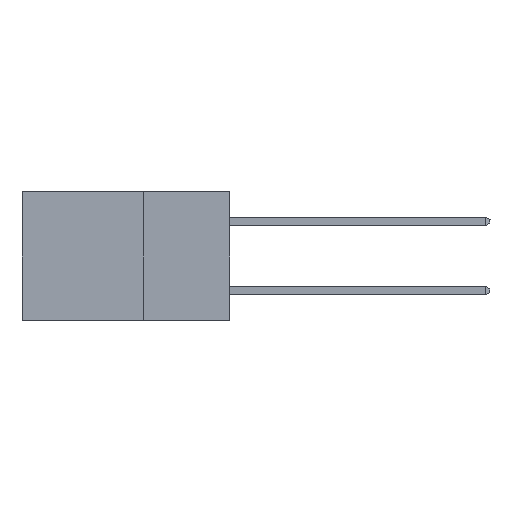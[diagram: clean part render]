
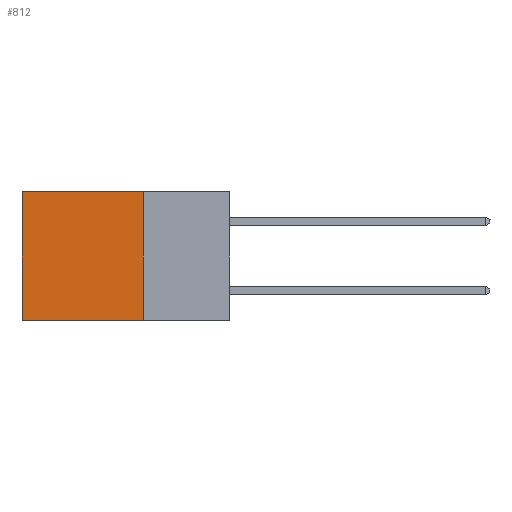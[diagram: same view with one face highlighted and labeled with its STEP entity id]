
A CAD part, left-side view. The second image highlights one B-rep face of the part: STEP entity #812.
In plain terms, the highlighted planar face has unit normal (-1, 0, 0).
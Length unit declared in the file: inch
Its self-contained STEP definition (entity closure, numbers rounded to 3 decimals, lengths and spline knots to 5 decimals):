
#155 = AXIS2_PLACEMENT_3D ( 'NONE', #5176, #6276, #11299 ) ;
#812 = ADVANCED_FACE ( 'NONE', ( #1641 ), #8886, .F. ) ;
#845 = ORIENTED_EDGE ( 'NONE', *, *, #6398, .T. ) ;
#1244 = CARTESIAN_POINT ( 'NONE',  ( 0.2615, 0.25, -0.37 ) ) ;
#1265 = VECTOR ( 'NONE', #4782, 39.37008 ) ;
#1641 = FACE_OUTER_BOUND ( 'NONE', #13665, .T. ) ;
#1705 = CARTESIAN_POINT ( 'NONE',  ( 0.2615, 0.6, -0.37 ) ) ;
#1787 = VERTEX_POINT ( 'NONE', #9597 ) ;
#1824 = LINE ( 'NONE', #1244, #1265 ) ;
#2248 = ORIENTED_EDGE ( 'NONE', *, *, #15168, .T. ) ;
#2853 = VERTEX_POINT ( 'NONE', #4912 ) ;
#3086 = DIRECTION ( 'NONE',  ( 0., 1., 0. ) ) ;
#3244 = CARTESIAN_POINT ( 'NONE',  ( 0.2615, 0.25, -0.37 ) ) ;
#3305 = VECTOR ( 'NONE', #6495, 39.37008 ) ;
#3324 = LINE ( 'NONE', #15288, #11066 ) ;
#3363 = CARTESIAN_POINT ( 'NONE',  ( 0.2615, 0.25, 0. ) ) ;
#4782 = DIRECTION ( 'NONE',  ( 0., 0., -1. ) ) ;
#4912 = CARTESIAN_POINT ( 'NONE',  ( 0.2615, 0.6, -0.37 ) ) ;
#5126 = EDGE_CURVE ( 'NONE', #6088, #2853, #5587, .T. ) ;
#5176 = CARTESIAN_POINT ( 'NONE',  ( 0.2615, 0.25, -0.37 ) ) ;
#5587 = LINE ( 'NONE', #3244, #8245 ) ;
#6088 = VERTEX_POINT ( 'NONE', #9247 ) ;
#6276 = DIRECTION ( 'NONE',  ( 1., 0., 0. ) ) ;
#6398 = EDGE_CURVE ( 'NONE', #13326, #1787, #3324, .T. ) ;
#6495 = DIRECTION ( 'NONE',  ( 0., 0., -1. ) ) ;
#8245 = VECTOR ( 'NONE', #3086, 39.37008 ) ;
#8886 = PLANE ( 'NONE',  #155 ) ;
#9247 = CARTESIAN_POINT ( 'NONE',  ( 0.2615, 0.25, -0.37 ) ) ;
#9597 = CARTESIAN_POINT ( 'NONE',  ( 0.2615, 0.6, 0. ) ) ;
#9731 = LINE ( 'NONE', #1705, #3305 ) ;
#11066 = VECTOR ( 'NONE', #12883, 39.37008 ) ;
#11299 = DIRECTION ( 'NONE',  ( 0., 0., -1. ) ) ;
#12404 = ORIENTED_EDGE ( 'NONE', *, *, #15025, .F. ) ;
#12883 = DIRECTION ( 'NONE',  ( 0., 1., 0. ) ) ;
#13326 = VERTEX_POINT ( 'NONE', #3363 ) ;
#13665 = EDGE_LOOP ( 'NONE', ( #2248, #13733, #12404, #845 ) ) ;
#13733 = ORIENTED_EDGE ( 'NONE', *, *, #5126, .F. ) ;
#15025 = EDGE_CURVE ( 'NONE', #13326, #6088, #1824, .T. ) ;
#15168 = EDGE_CURVE ( 'NONE', #1787, #2853, #9731, .T. ) ;
#15288 = CARTESIAN_POINT ( 'NONE',  ( 0.2615, 0.25, 0. ) ) ;
